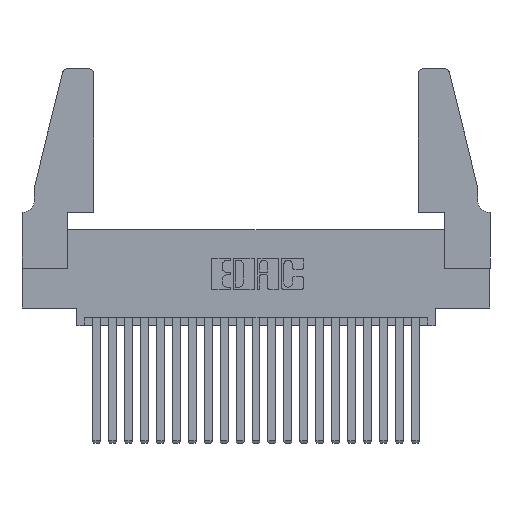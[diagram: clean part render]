
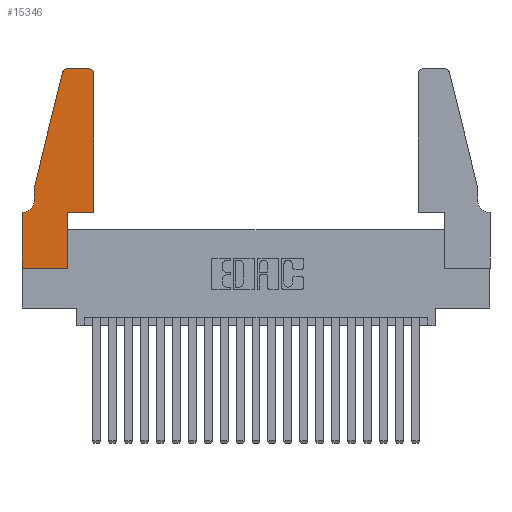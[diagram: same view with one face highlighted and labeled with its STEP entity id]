
A CAD part, top view. The second image highlights one B-rep face of the part: STEP entity #15346.
In plain terms, the highlighted planar face has unit normal (0, 0, 1).
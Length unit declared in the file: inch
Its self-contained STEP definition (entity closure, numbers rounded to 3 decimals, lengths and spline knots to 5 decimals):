
#234 = CARTESIAN_POINT ( 'NONE',  ( 0.0055, 0.42, 0.37 ) ) ;
#282 = VERTEX_POINT ( 'NONE', #3244 ) ;
#322 = VERTEX_POINT ( 'NONE', #10026 ) ;
#347 = EDGE_CURVE ( 'NONE', #7663, #563, #8594, .T. ) ;
#400 = CARTESIAN_POINT ( 'NONE',  ( 0., 0., 0.37 ) ) ;
#563 = VERTEX_POINT ( 'NONE', #12594 ) ;
#750 = DIRECTION ( 'NONE',  ( 0., 0., 1. ) ) ;
#817 = DIRECTION ( 'NONE',  ( 1., 0., 0. ) ) ;
#1006 = VERTEX_POINT ( 'NONE', #2945 ) ;
#1154 = VECTOR ( 'NONE', #21334, 39.37008 ) ;
#1230 = VECTOR ( 'NONE', #12658, 39.37008 ) ;
#1634 = CARTESIAN_POINT ( 'NONE',  ( 0.4505, 0.35, 0.37 ) ) ;
#1877 = DIRECTION ( 'NONE',  ( 0., 0., -1. ) ) ;
#1908 = DIRECTION ( 'NONE',  ( 0., -1., 0. ) ) ;
#1927 = EDGE_CURVE ( 'NONE', #2830, #7663, #3967, .T. ) ;
#2015 = FACE_OUTER_BOUND ( 'NONE', #20708, .T. ) ;
#2313 = LINE ( 'NONE', #17040, #2881 ) ;
#2398 = CARTESIAN_POINT ( 'NONE',  ( 0.0755, 0.35, 0.37 ) ) ;
#2437 = EDGE_CURVE ( 'NONE', #17512, #5589, #2313, .T. ) ;
#2830 = VERTEX_POINT ( 'NONE', #19666 ) ;
#2881 = VECTOR ( 'NONE', #7276, 39.37008 ) ;
#2913 = CARTESIAN_POINT ( 'NONE',  ( 0.2865, 0., 0.37 ) ) ;
#2945 = CARTESIAN_POINT ( 'NONE',  ( 0.0755, 0.5, 0.37 ) ) ;
#3244 = CARTESIAN_POINT ( 'NONE',  ( 0.4205, 1.25, 0.37 ) ) ;
#3540 = EDGE_CURVE ( 'NONE', #5589, #20587, #12870, .T. ) ;
#3967 = CIRCLE ( 'NONE', #19376, 0.07 ) ;
#4599 = AXIS2_PLACEMENT_3D ( 'NONE', #18977, #10874, #817 ) ;
#5152 = VERTEX_POINT ( 'NONE', #400 ) ;
#5521 = CARTESIAN_POINT ( 'NONE',  ( 0.2865, 0.35, 0.37 ) ) ;
#5589 = VERTEX_POINT ( 'NONE', #19647 ) ;
#5704 = ORIENTED_EDGE ( 'NONE', *, *, #11940, .T. ) ;
#5766 = ORIENTED_EDGE ( 'NONE', *, *, #16984, .T. ) ;
#5794 = VECTOR ( 'NONE', #1908, 39.37008 ) ;
#6285 = VECTOR ( 'NONE', #11349, 39.37008 ) ;
#6644 = CARTESIAN_POINT ( 'NONE',  ( 0.4505, 1.22, 0.37 ) ) ;
#6792 = CIRCLE ( 'NONE', #18960, 0.03 ) ;
#7276 = DIRECTION ( 'NONE',  ( 1., 0., 0. ) ) ;
#7326 = DIRECTION ( 'NONE',  ( -1., 0., 0. ) ) ;
#7468 = VECTOR ( 'NONE', #20283, 39.37008 ) ;
#7578 = PLANE ( 'NONE',  #4599 ) ;
#7663 = VERTEX_POINT ( 'NONE', #11898 ) ;
#8158 = EDGE_CURVE ( 'NONE', #20587, #282, #15120, .T. ) ;
#8475 = VERTEX_POINT ( 'NONE', #10117 ) ;
#8529 = CARTESIAN_POINT ( 'NONE',  ( 0.0755, 0.5, 0.37 ) ) ;
#8594 = LINE ( 'NONE', #2398, #16706 ) ;
#8609 = VECTOR ( 'NONE', #14347, 39.37008 ) ;
#9140 = LINE ( 'NONE', #11095, #8609 ) ;
#9269 = ORIENTED_EDGE ( 'NONE', *, *, #14743, .T. ) ;
#9298 = CARTESIAN_POINT ( 'NONE',  ( 0.4205, 1.22, 0.37 ) ) ;
#9638 = VERTEX_POINT ( 'NONE', #2913 ) ;
#9779 = ORIENTED_EDGE ( 'NONE', *, *, #2437, .T. ) ;
#9786 = ORIENTED_EDGE ( 'NONE', *, *, #1927, .T. ) ;
#10026 = CARTESIAN_POINT ( 'NONE',  ( 0.25487, 1.22718, 0.37 ) ) ;
#10117 = CARTESIAN_POINT ( 'NONE',  ( 0.284, 1.25, 0.37 ) ) ;
#10239 = CARTESIAN_POINT ( 'NONE',  ( 0., 0., 0.37 ) ) ;
#10304 = LINE ( 'NONE', #18646, #7468 ) ;
#10650 = LINE ( 'NONE', #14517, #6285 ) ;
#10832 = CARTESIAN_POINT ( 'NONE',  ( 0.284, 1.22, 0.37 ) ) ;
#10874 = DIRECTION ( 'NONE',  ( 0., 0., 1. ) ) ;
#10914 = DIRECTION ( 'NONE',  ( 1., 0., 0. ) ) ;
#11095 = CARTESIAN_POINT ( 'NONE',  ( 0.2865, 0.35, 0.37 ) ) ;
#11173 = LINE ( 'NONE', #14272, #1230 ) ;
#11174 = VECTOR ( 'NONE', #18252, 39.37008 ) ;
#11349 = DIRECTION ( 'NONE',  ( 1., 0., 0. ) ) ;
#11898 = CARTESIAN_POINT ( 'NONE',  ( 0.0055, 0.35, 0.37 ) ) ;
#11940 = EDGE_CURVE ( 'NONE', #1006, #2830, #15489, .T. ) ;
#11972 = EDGE_CURVE ( 'NONE', #563, #5152, #14450, .T. ) ;
#12396 = EDGE_CURVE ( 'NONE', #5152, #9638, #10650, .T. ) ;
#12440 = ORIENTED_EDGE ( 'NONE', *, *, #13513, .T. ) ;
#12457 = DIRECTION ( 'NONE',  ( 1., 0., 0. ) ) ;
#12492 = ORIENTED_EDGE ( 'NONE', *, *, #14615, .T. ) ;
#12594 = CARTESIAN_POINT ( 'NONE',  ( 0., 0.35, 0.37 ) ) ;
#12658 = DIRECTION ( 'NONE',  ( -1., 0., 0. ) ) ;
#12753 = AXIS2_PLACEMENT_3D ( 'NONE', #9298, #20635, #10914 ) ;
#12870 = LINE ( 'NONE', #1634, #1154 ) ;
#12988 = ORIENTED_EDGE ( 'NONE', *, *, #12396, .T. ) ;
#13513 = EDGE_CURVE ( 'NONE', #282, #8475, #11173, .T. ) ;
#13806 = ORIENTED_EDGE ( 'NONE', *, *, #3540, .T. ) ;
#14162 = ORIENTED_EDGE ( 'NONE', *, *, #8158, .T. ) ;
#14272 = CARTESIAN_POINT ( 'NONE',  ( 0.2605, 1.25, 0.37 ) ) ;
#14347 = DIRECTION ( 'NONE',  ( 0., 1., 0. ) ) ;
#14450 = LINE ( 'NONE', #10239, #5794 ) ;
#14517 = CARTESIAN_POINT ( 'NONE',  ( 0., 0., 0.37 ) ) ;
#14615 = EDGE_CURVE ( 'NONE', #8475, #322, #6792, .T. ) ;
#14743 = EDGE_CURVE ( 'NONE', #9638, #17512, #9140, .T. ) ;
#15120 = CIRCLE ( 'NONE', #12753, 0.03 ) ;
#15346 = ADVANCED_FACE ( 'NONE', ( #2015 ), #7578, .T. ) ;
#15489 = LINE ( 'NONE', #8529, #11174 ) ;
#15773 = ORIENTED_EDGE ( 'NONE', *, *, #347, .T. ) ;
#16706 = VECTOR ( 'NONE', #7326, 39.37008 ) ;
#16984 = EDGE_CURVE ( 'NONE', #322, #1006, #10304, .T. ) ;
#17040 = CARTESIAN_POINT ( 'NONE',  ( 0.4505, 0.35, 0.37 ) ) ;
#17065 = ORIENTED_EDGE ( 'NONE', *, *, #11972, .T. ) ;
#17512 = VERTEX_POINT ( 'NONE', #5521 ) ;
#18252 = DIRECTION ( 'NONE',  ( 0., -1., 0. ) ) ;
#18646 = CARTESIAN_POINT ( 'NONE',  ( 0.0755, 0.5, 0.37 ) ) ;
#18960 = AXIS2_PLACEMENT_3D ( 'NONE', #10832, #750, #12457 ) ;
#18977 = CARTESIAN_POINT ( 'NONE',  ( 0., 0.35, 0.37 ) ) ;
#19376 = AXIS2_PLACEMENT_3D ( 'NONE', #234, #1877, #20057 ) ;
#19647 = CARTESIAN_POINT ( 'NONE',  ( 0.4505, 0.35, 0.37 ) ) ;
#19666 = CARTESIAN_POINT ( 'NONE',  ( 0.0755, 0.42, 0.37 ) ) ;
#20057 = DIRECTION ( 'NONE',  ( -1., 0., 0. ) ) ;
#20283 = DIRECTION ( 'NONE',  ( -0.239, -0.971, 0. ) ) ;
#20587 = VERTEX_POINT ( 'NONE', #6644 ) ;
#20635 = DIRECTION ( 'NONE',  ( 0., 0., 1. ) ) ;
#20708 = EDGE_LOOP ( 'NONE', ( #12440, #12492, #5766, #5704, #9786, #15773, #17065, #12988, #9269, #9779, #13806, #14162 ) ) ;
#21334 = DIRECTION ( 'NONE',  ( 0., 1., 0. ) ) ;
